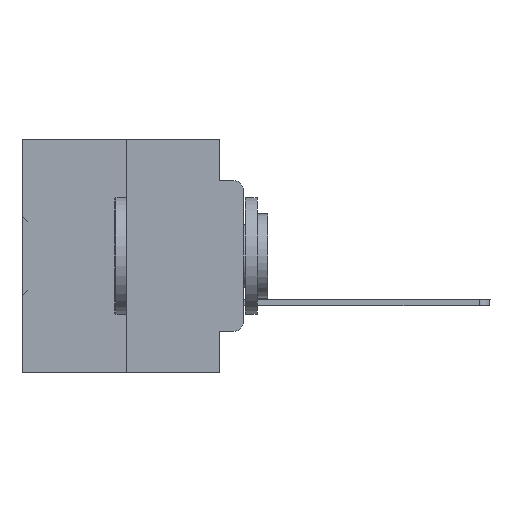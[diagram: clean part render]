
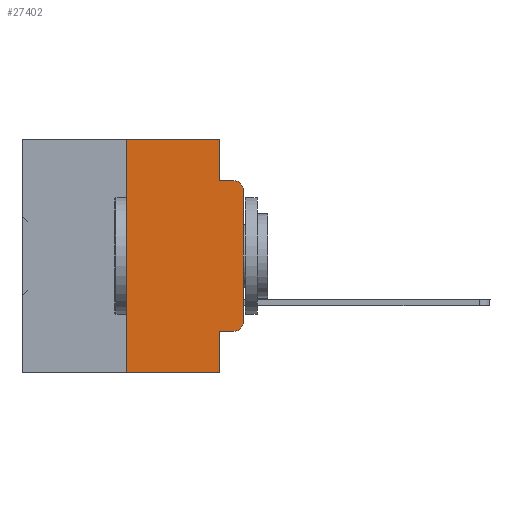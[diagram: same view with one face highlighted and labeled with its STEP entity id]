
A CAD part, left-side view. The second image highlights one B-rep face of the part: STEP entity #27402.
In plain terms, the highlighted planar face has unit normal (-1, 0, 0).
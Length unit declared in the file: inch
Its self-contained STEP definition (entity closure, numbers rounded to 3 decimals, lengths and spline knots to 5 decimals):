
#547 = ORIENTED_EDGE ( 'NONE', *, *, #23078, .F. ) ;
#1769 = VERTEX_POINT ( 'NONE', #35513 ) ;
#2161 = CARTESIAN_POINT ( 'NONE',  ( 0., 0.051, -0.5 ) ) ;
#2223 = ORIENTED_EDGE ( 'NONE', *, *, #9184, .F. ) ;
#2505 = VERTEX_POINT ( 'NONE', #22182 ) ;
#2808 = AXIS2_PLACEMENT_3D ( 'NONE', #19766, #34767, #20146 ) ;
#3292 = VECTOR ( 'NONE', #31585, 39.37008 ) ;
#4208 = ORIENTED_EDGE ( 'NONE', *, *, #26020, .T. ) ;
#4740 = ORIENTED_EDGE ( 'NONE', *, *, #9905, .F. ) ;
#4857 = CARTESIAN_POINT ( 'NONE',  ( 0., 0.25, 0. ) ) ;
#5773 = VECTOR ( 'NONE', #22619, 39.37008 ) ;
#6063 = EDGE_CURVE ( 'NONE', #2505, #15122, #12031, .T. ) ;
#7107 = AXIS2_PLACEMENT_3D ( 'NONE', #23801, #17972, #29283 ) ;
#7874 = FACE_OUTER_BOUND ( 'NONE', #22984, .T. ) ;
#8429 = VERTEX_POINT ( 'NONE', #2161 ) ;
#8877 = ORIENTED_EDGE ( 'NONE', *, *, #36287, .T. ) ;
#9184 = EDGE_CURVE ( 'NONE', #2505, #8429, #15731, .T. ) ;
#9368 = LINE ( 'NONE', #33156, #20940 ) ;
#9905 = EDGE_CURVE ( 'NONE', #1769, #22067, #22003, .T. ) ;
#10100 = DIRECTION ( 'NONE',  ( 0., 0., -1. ) ) ;
#11749 = CARTESIAN_POINT ( 'NONE',  ( 0., 0.25, -0.5 ) ) ;
#12031 = LINE ( 'NONE', #16602, #5773 ) ;
#14493 = DIRECTION ( 'NONE',  ( 0., -1., 0. ) ) ;
#14683 = ORIENTED_EDGE ( 'NONE', *, *, #32839, .F. ) ;
#14733 = CARTESIAN_POINT ( 'NONE',  ( 0., 0.02, -0.4115 ) ) ;
#15122 = VERTEX_POINT ( 'NONE', #14733 ) ;
#15505 = EDGE_CURVE ( 'NONE', #36438, #1769, #9368, .T. ) ;
#15677 = CARTESIAN_POINT ( 'NONE',  ( 0., 0., 0. ) ) ;
#15731 = LINE ( 'NONE', #24680, #31890 ) ;
#16602 = CARTESIAN_POINT ( 'NONE',  ( 0., 0.051, -0.4115 ) ) ;
#17039 = ORIENTED_EDGE ( 'NONE', *, *, #6063, .T. ) ;
#17284 = CARTESIAN_POINT ( 'NONE',  ( 0., 0.473, 0. ) ) ;
#17418 = CARTESIAN_POINT ( 'NONE',  ( 0., 0.473, -0.5 ) ) ;
#17704 = VECTOR ( 'NONE', #35207, 39.37008 ) ;
#17921 = CARTESIAN_POINT ( 'NONE',  ( 0., 0., -0.3915 ) ) ;
#17972 = DIRECTION ( 'NONE',  ( -1., 0., 0. ) ) ;
#18060 = ORIENTED_EDGE ( 'NONE', *, *, #15505, .F. ) ;
#19228 = DIRECTION ( 'NONE',  ( 0., 0., -1. ) ) ;
#19243 = VERTEX_POINT ( 'NONE', #17921 ) ;
#19766 = CARTESIAN_POINT ( 'NONE',  ( 0., 0.473, 0. ) ) ;
#20071 = VECTOR ( 'NONE', #14493, 39.37008 ) ;
#20146 = DIRECTION ( 'NONE',  ( 0., 0., -1. ) ) ;
#20332 = CARTESIAN_POINT ( 'NONE',  ( 0., 0.25, 0. ) ) ;
#20341 = LINE ( 'NONE', #17418, #20071 ) ;
#20583 = EDGE_CURVE ( 'NONE', #30332, #8429, #20341, .T. ) ;
#20940 = VECTOR ( 'NONE', #36244, 39.37008 ) ;
#22003 = LINE ( 'NONE', #31186, #3292 ) ;
#22067 = VERTEX_POINT ( 'NONE', #27563 ) ;
#22182 = CARTESIAN_POINT ( 'NONE',  ( 0., 0.051, -0.4115 ) ) ;
#22569 = DIRECTION ( 'NONE',  ( -1., 0., 0. ) ) ;
#22619 = DIRECTION ( 'NONE',  ( 0., -1., 0. ) ) ;
#22984 = EDGE_LOOP ( 'NONE', ( #4208, #8877, #4740, #18060, #547, #14683, #23420, #2223, #17039, #28537 ) ) ;
#23078 = EDGE_CURVE ( 'NONE', #38356, #36438, #32107, .T. ) ;
#23295 = AXIS2_PLACEMENT_3D ( 'NONE', #30780, #22569, #10100 ) ;
#23420 = ORIENTED_EDGE ( 'NONE', *, *, #20583, .T. ) ;
#23801 = CARTESIAN_POINT ( 'NONE',  ( 0., 0.02, -0.1085 ) ) ;
#24539 = CIRCLE ( 'NONE', #23295, 0.02 ) ;
#24680 = CARTESIAN_POINT ( 'NONE',  ( 0., 0.051, 0. ) ) ;
#25182 = EDGE_CURVE ( 'NONE', #15122, #19243, #24539, .T. ) ;
#26020 = EDGE_CURVE ( 'NONE', #19243, #35504, #31074, .T. ) ;
#27003 = CIRCLE ( 'NONE', #7107, 0.02 ) ;
#27134 = DIRECTION ( 'NONE',  ( 0., 0., 1. ) ) ;
#27402 = ADVANCED_FACE ( 'NONE', ( #7874 ), #34571, .F. ) ;
#27495 = CARTESIAN_POINT ( 'NONE',  ( 0., 0.051, 0. ) ) ;
#27563 = CARTESIAN_POINT ( 'NONE',  ( 0., 0.02, -0.0885 ) ) ;
#28341 = VECTOR ( 'NONE', #34361, 39.37008 ) ;
#28537 = ORIENTED_EDGE ( 'NONE', *, *, #25182, .T. ) ;
#29097 = CARTESIAN_POINT ( 'NONE',  ( 0., 0., -0.1085 ) ) ;
#29283 = DIRECTION ( 'NONE',  ( 0., 0., -1. ) ) ;
#29677 = LINE ( 'NONE', #20332, #32315 ) ;
#30332 = VERTEX_POINT ( 'NONE', #11749 ) ;
#30780 = CARTESIAN_POINT ( 'NONE',  ( 0., 0.02, -0.3915 ) ) ;
#31074 = LINE ( 'NONE', #15677, #28341 ) ;
#31186 = CARTESIAN_POINT ( 'NONE',  ( 0., 0.051, -0.0885 ) ) ;
#31585 = DIRECTION ( 'NONE',  ( 0., -1., 0. ) ) ;
#31890 = VECTOR ( 'NONE', #19228, 39.37008 ) ;
#32107 = LINE ( 'NONE', #17284, #17704 ) ;
#32315 = VECTOR ( 'NONE', #27134, 39.37008 ) ;
#32839 = EDGE_CURVE ( 'NONE', #30332, #38356, #29677, .T. ) ;
#33156 = CARTESIAN_POINT ( 'NONE',  ( 0., 0.051, 0. ) ) ;
#34361 = DIRECTION ( 'NONE',  ( 0., 0., 1. ) ) ;
#34571 = PLANE ( 'NONE',  #2808 ) ;
#34767 = DIRECTION ( 'NONE',  ( 1., 0., 0. ) ) ;
#35207 = DIRECTION ( 'NONE',  ( 0., -1., 0. ) ) ;
#35504 = VERTEX_POINT ( 'NONE', #29097 ) ;
#35513 = CARTESIAN_POINT ( 'NONE',  ( 0., 0.051, -0.0885 ) ) ;
#36244 = DIRECTION ( 'NONE',  ( 0., 0., -1. ) ) ;
#36287 = EDGE_CURVE ( 'NONE', #35504, #22067, #27003, .T. ) ;
#36438 = VERTEX_POINT ( 'NONE', #27495 ) ;
#38356 = VERTEX_POINT ( 'NONE', #4857 ) ;
